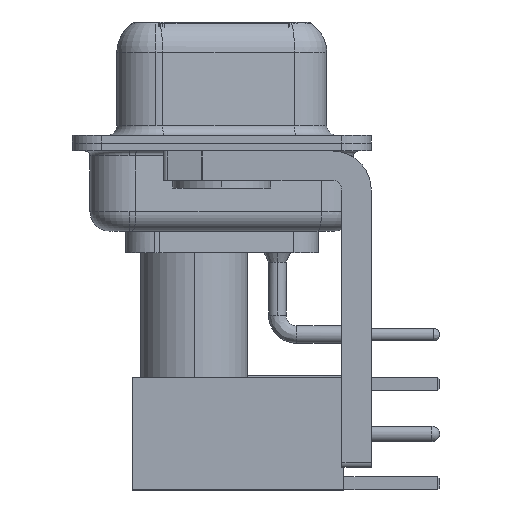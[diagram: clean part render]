
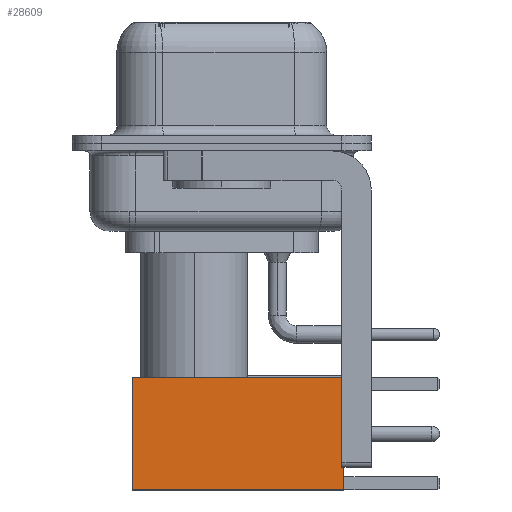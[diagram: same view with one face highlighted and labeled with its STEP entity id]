
A CAD part, left-side view. The second image highlights one B-rep face of the part: STEP entity #28609.
In plain terms, the highlighted face is planar.
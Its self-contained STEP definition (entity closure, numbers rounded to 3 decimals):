
#710 = ORIENTED_EDGE ( 'NONE', *, *, #6136, .F. ) ;
#1861 = ORIENTED_EDGE ( 'NONE', *, *, #25099, .T. ) ;
#2790 = FACE_OUTER_BOUND ( 'NONE', #4124, .T. ) ;
#4124 = EDGE_LOOP ( 'NONE', ( #1861, #31647, #26745, #710 ) ) ;
#5444 = LINE ( 'NONE', #28253, #12444 ) ;
#6136 = EDGE_CURVE ( 'NONE', #27350, #26151, #24556, .T. ) ;
#6631 = VERTEX_POINT ( 'NONE', #19350 ) ;
#8998 = LINE ( 'NONE', #30057, #15522 ) ;
#9187 = DIRECTION ( 'NONE',  ( 0., 0., -1. ) ) ;
#9996 = DIRECTION ( 'NONE',  ( -1., 0., 0. ) ) ;
#10360 = VECTOR ( 'NONE', #25766, 1000. ) ;
#11228 = CARTESIAN_POINT ( 'NONE',  ( 2.875, 2.875, 0. ) ) ;
#11419 = DIRECTION ( 'NONE',  ( 0., 1., 0. ) ) ;
#12444 = VECTOR ( 'NONE', #34762, 1000. ) ;
#14487 = DIRECTION ( 'NONE',  ( 0., 0., 1. ) ) ;
#15522 = VECTOR ( 'NONE', #9187, 1000. ) ;
#16225 = VECTOR ( 'NONE', #9996, 1000. ) ;
#16981 = PLANE ( 'NONE',  #21823 ) ;
#19350 = CARTESIAN_POINT ( 'NONE',  ( -2.875, 2.875, 0. ) ) ;
#19850 = CARTESIAN_POINT ( 'NONE',  ( 2.875, 2.875, 10.82 ) ) ;
#20159 = EDGE_CURVE ( 'NONE', #26151, #6631, #24990, .T. ) ;
#21823 = AXIS2_PLACEMENT_3D ( 'NONE', #11228, #11419, #14487 ) ;
#24556 = LINE ( 'NONE', #36251, #16225 ) ;
#24737 = EDGE_CURVE ( 'NONE', #30191, #6631, #5444, .T. ) ;
#24990 = LINE ( 'NONE', #25384, #10360 ) ;
#25099 = EDGE_CURVE ( 'NONE', #27350, #30191, #8998, .T. ) ;
#25384 = CARTESIAN_POINT ( 'NONE',  ( -2.875, 2.875, 0. ) ) ;
#25766 = DIRECTION ( 'NONE',  ( 0., 0., -1. ) ) ;
#26151 = VERTEX_POINT ( 'NONE', #30479 ) ;
#26745 = ORIENTED_EDGE ( 'NONE', *, *, #20159, .F. ) ;
#27350 = VERTEX_POINT ( 'NONE', #19850 ) ;
#28253 = CARTESIAN_POINT ( 'NONE',  ( 0., 2.875, 0. ) ) ;
#28609 = ADVANCED_FACE ( 'NONE', ( #2790 ), #16981, .T. ) ;
#30057 = CARTESIAN_POINT ( 'NONE',  ( 2.875, 2.875, 0. ) ) ;
#30191 = VERTEX_POINT ( 'NONE', #34009 ) ;
#30479 = CARTESIAN_POINT ( 'NONE',  ( -2.875, 2.875, 10.82 ) ) ;
#31647 = ORIENTED_EDGE ( 'NONE', *, *, #24737, .T. ) ;
#34009 = CARTESIAN_POINT ( 'NONE',  ( 2.875, 2.875, 0. ) ) ;
#34762 = DIRECTION ( 'NONE',  ( -1., 0., 0. ) ) ;
#36251 = CARTESIAN_POINT ( 'NONE',  ( 0., 2.875, 10.82 ) ) ;
